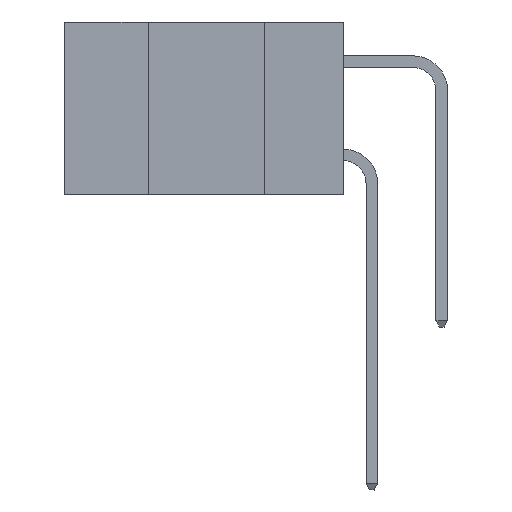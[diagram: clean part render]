
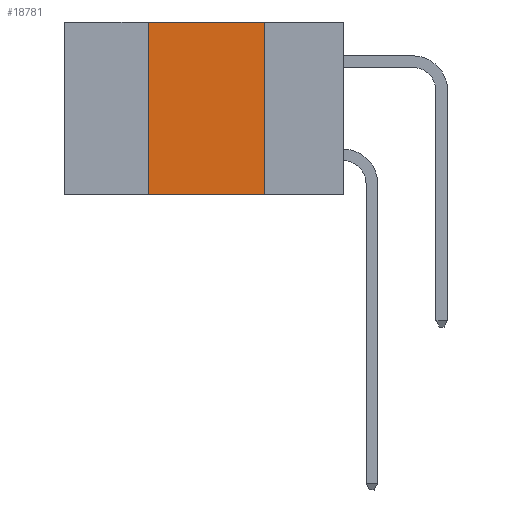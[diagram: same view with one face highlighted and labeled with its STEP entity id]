
A CAD part, left-side view. The second image highlights one B-rep face of the part: STEP entity #18781.
In plain terms, the highlighted planar face has unit normal (-1, 0, 0).
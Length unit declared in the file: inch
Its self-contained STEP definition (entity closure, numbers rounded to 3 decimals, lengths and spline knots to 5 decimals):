
#155 = VERTEX_POINT ( 'NONE', #10838 ) ;
#562 = CARTESIAN_POINT ( 'NONE',  ( 0., 0.42, -0.37 ) ) ;
#1677 = LINE ( 'NONE', #8568, #14416 ) ;
#2760 = VERTEX_POINT ( 'NONE', #9908 ) ;
#4535 = LINE ( 'NONE', #13028, #17854 ) ;
#4926 = ORIENTED_EDGE ( 'NONE', *, *, #18911, .F. ) ;
#6399 = DIRECTION ( 'NONE',  ( 0., -1., 0. ) ) ;
#7234 = CARTESIAN_POINT ( 'NONE',  ( 0., 0.17, -0.37 ) ) ;
#8452 = CARTESIAN_POINT ( 'NONE',  ( 0., 0.42, -0.37 ) ) ;
#8568 = CARTESIAN_POINT ( 'NONE',  ( 0., 0.6, -0.37 ) ) ;
#9342 = DIRECTION ( 'NONE',  ( 0., 0., 1. ) ) ;
#9381 = EDGE_LOOP ( 'NONE', ( #25737, #4926, #28122, #26193 ) ) ;
#9908 = CARTESIAN_POINT ( 'NONE',  ( 0., 0.17, 0. ) ) ;
#10314 = LINE ( 'NONE', #27929, #23850 ) ;
#10838 = CARTESIAN_POINT ( 'NONE',  ( 0., 0.42, 0. ) ) ;
#10866 = DIRECTION ( 'NONE',  ( 0., 0., -1. ) ) ;
#11719 = VERTEX_POINT ( 'NONE', #8452 ) ;
#13028 = CARTESIAN_POINT ( 'NONE',  ( 0., 0.6, 0. ) ) ;
#13479 = EDGE_CURVE ( 'NONE', #11719, #24558, #1677, .T. ) ;
#14416 = VECTOR ( 'NONE', #6399, 39.37008 ) ;
#15394 = VECTOR ( 'NONE', #9342, 39.37008 ) ;
#16937 = AXIS2_PLACEMENT_3D ( 'NONE', #19550, #21709, #10866 ) ;
#17666 = DIRECTION ( 'NONE',  ( 0., -1., 0. ) ) ;
#17854 = VECTOR ( 'NONE', #17666, 39.37008 ) ;
#18558 = DIRECTION ( 'NONE',  ( 0., 0., -1. ) ) ;
#18711 = EDGE_CURVE ( 'NONE', #2760, #24558, #10314, .T. ) ;
#18781 = ADVANCED_FACE ( 'NONE', ( #26185 ), #23876, .F. ) ;
#18911 = EDGE_CURVE ( 'NONE', #155, #2760, #4535, .T. ) ;
#19550 = CARTESIAN_POINT ( 'NONE',  ( 0., 0.6, 0. ) ) ;
#20335 = EDGE_CURVE ( 'NONE', #11719, #155, #22631, .T. ) ;
#21709 = DIRECTION ( 'NONE',  ( 1., 0., 0. ) ) ;
#22631 = LINE ( 'NONE', #562, #15394 ) ;
#23850 = VECTOR ( 'NONE', #18558, 39.37008 ) ;
#23876 = PLANE ( 'NONE',  #16937 ) ;
#24558 = VERTEX_POINT ( 'NONE', #7234 ) ;
#25737 = ORIENTED_EDGE ( 'NONE', *, *, #18711, .F. ) ;
#26185 = FACE_OUTER_BOUND ( 'NONE', #9381, .T. ) ;
#26193 = ORIENTED_EDGE ( 'NONE', *, *, #13479, .T. ) ;
#27929 = CARTESIAN_POINT ( 'NONE',  ( 0., 0.17, -0.37 ) ) ;
#28122 = ORIENTED_EDGE ( 'NONE', *, *, #20335, .F. ) ;
